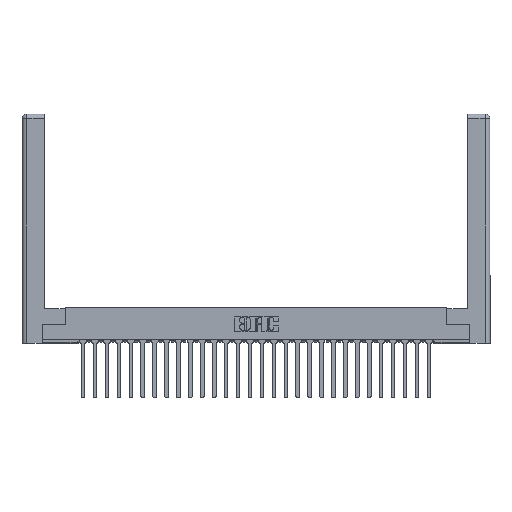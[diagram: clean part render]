
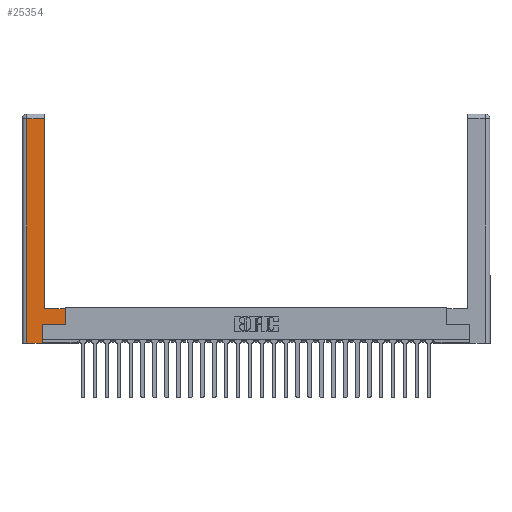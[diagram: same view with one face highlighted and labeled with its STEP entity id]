
A CAD part, top view. The second image highlights one B-rep face of the part: STEP entity #25354.
In plain terms, the highlighted planar face has unit normal (0, 0, 1).
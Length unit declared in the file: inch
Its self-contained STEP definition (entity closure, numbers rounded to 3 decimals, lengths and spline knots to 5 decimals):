
#52 = VERTEX_POINT ( 'NONE', #24786 ) ;
#271 = CARTESIAN_POINT ( 'NONE',  ( 0.565, 0.245, 0. ) ) ;
#690 = VECTOR ( 'NONE', #3820, 39.37008 ) ;
#860 = DIRECTION ( 'NONE',  ( 0., 0., -1. ) ) ;
#1262 = ORIENTED_EDGE ( 'NONE', *, *, #14291, .T. ) ;
#1794 = ORIENTED_EDGE ( 'NONE', *, *, #5405, .T. ) ;
#1937 = VECTOR ( 'NONE', #23098, 39.37008 ) ;
#2169 = CARTESIAN_POINT ( 'NONE',  ( 0.565, 0.45, 0. ) ) ;
#2678 = VECTOR ( 'NONE', #24976, 39.37008 ) ;
#2808 = DIRECTION ( 'NONE',  ( 0., 1., 0. ) ) ;
#3031 = VECTOR ( 'NONE', #5175, 39.37008 ) ;
#3820 = DIRECTION ( 'NONE',  ( 1., 0., 0. ) ) ;
#4537 = CARTESIAN_POINT ( 'NONE',  ( 0.565, 0.245, 0. ) ) ;
#4608 = AXIS2_PLACEMENT_3D ( 'NONE', #16785, #860, #5310 ) ;
#4764 = CARTESIAN_POINT ( 'NONE',  ( 0.295, 3., 0. ) ) ;
#4969 = CARTESIAN_POINT ( 'NONE',  ( 0.0615, 2.94, 0. ) ) ;
#5010 = PLANE ( 'NONE',  #4608 ) ;
#5175 = DIRECTION ( 'NONE',  ( 0., 1., 0. ) ) ;
#5310 = DIRECTION ( 'NONE',  ( -1., 0., 0. ) ) ;
#5324 = EDGE_CURVE ( 'NONE', #21354, #5573, #17789, .T. ) ;
#5362 = VERTEX_POINT ( 'NONE', #10994 ) ;
#5405 = EDGE_CURVE ( 'NONE', #10298, #19032, #8087, .T. ) ;
#5573 = VERTEX_POINT ( 'NONE', #26374 ) ;
#5722 = EDGE_CURVE ( 'NONE', #5362, #13700, #21044, .T. ) ;
#6211 = CARTESIAN_POINT ( 'NONE',  ( 0.265, 0.245, 0. ) ) ;
#6610 = ORIENTED_EDGE ( 'NONE', *, *, #22366, .T. ) ;
#7344 = DIRECTION ( 'NONE',  ( -1., 0., 0. ) ) ;
#7963 = CARTESIAN_POINT ( 'NONE',  ( 0.265, 0., 0. ) ) ;
#8087 = LINE ( 'NONE', #16650, #3031 ) ;
#8960 = LINE ( 'NONE', #4764, #25109 ) ;
#10219 = EDGE_CURVE ( 'NONE', #13700, #21354, #27343, .T. ) ;
#10298 = VERTEX_POINT ( 'NONE', #4537 ) ;
#10642 = CARTESIAN_POINT ( 'NONE',  ( 0.0615, 0., 0. ) ) ;
#10994 = CARTESIAN_POINT ( 'NONE',  ( 0.0615, 2.94, 0. ) ) ;
#11198 = DIRECTION ( 'NONE',  ( 0., 1., 0. ) ) ;
#11674 = EDGE_CURVE ( 'NONE', #12180, #5362, #11866, .T. ) ;
#11808 = ORIENTED_EDGE ( 'NONE', *, *, #10219, .T. ) ;
#11866 = LINE ( 'NONE', #4969, #18661 ) ;
#12180 = VERTEX_POINT ( 'NONE', #21714 ) ;
#13198 = CARTESIAN_POINT ( 'NONE',  ( 0.265, 0., 0. ) ) ;
#13452 = CARTESIAN_POINT ( 'NONE',  ( 0.295, 0.45, 0. ) ) ;
#13700 = VERTEX_POINT ( 'NONE', #10642 ) ;
#13899 = VECTOR ( 'NONE', #11198, 39.37008 ) ;
#14291 = EDGE_CURVE ( 'NONE', #5573, #10298, #23856, .T. ) ;
#15644 = CARTESIAN_POINT ( 'NONE',  ( 0.0615, 0., 0. ) ) ;
#16650 = CARTESIAN_POINT ( 'NONE',  ( 0.565, 0.45, 0. ) ) ;
#16785 = CARTESIAN_POINT ( 'NONE',  ( 0., 0., 0. ) ) ;
#17789 = LINE ( 'NONE', #6211, #13899 ) ;
#18661 = VECTOR ( 'NONE', #7344, 39.37008 ) ;
#19032 = VERTEX_POINT ( 'NONE', #2169 ) ;
#20717 = DIRECTION ( 'NONE',  ( 1., 0., 0. ) ) ;
#21044 = LINE ( 'NONE', #15644, #1937 ) ;
#21354 = VERTEX_POINT ( 'NONE', #7963 ) ;
#21714 = CARTESIAN_POINT ( 'NONE',  ( 0.295, 2.94, 0. ) ) ;
#21735 = EDGE_LOOP ( 'NONE', ( #28416, #27390, #23481, #11808, #24596, #1262, #1794, #6610 ) ) ;
#22366 = EDGE_CURVE ( 'NONE', #19032, #52, #24293, .T. ) ;
#23098 = DIRECTION ( 'NONE',  ( 0., -1., 0. ) ) ;
#23481 = ORIENTED_EDGE ( 'NONE', *, *, #5722, .T. ) ;
#23856 = LINE ( 'NONE', #271, #25681 ) ;
#24293 = LINE ( 'NONE', #13452, #2678 ) ;
#24593 = FACE_OUTER_BOUND ( 'NONE', #21735, .T. ) ;
#24596 = ORIENTED_EDGE ( 'NONE', *, *, #5324, .T. ) ;
#24786 = CARTESIAN_POINT ( 'NONE',  ( 0.295, 0.45, 0. ) ) ;
#24976 = DIRECTION ( 'NONE',  ( -1., 0., 0. ) ) ;
#25109 = VECTOR ( 'NONE', #2808, 39.37008 ) ;
#25354 = ADVANCED_FACE ( 'NONE', ( #24593 ), #5010, .F. ) ;
#25681 = VECTOR ( 'NONE', #20717, 39.37008 ) ;
#26374 = CARTESIAN_POINT ( 'NONE',  ( 0.265, 0.245, 0. ) ) ;
#27343 = LINE ( 'NONE', #13198, #690 ) ;
#27390 = ORIENTED_EDGE ( 'NONE', *, *, #11674, .T. ) ;
#28134 = EDGE_CURVE ( 'NONE', #52, #12180, #8960, .T. ) ;
#28416 = ORIENTED_EDGE ( 'NONE', *, *, #28134, .T. ) ;
